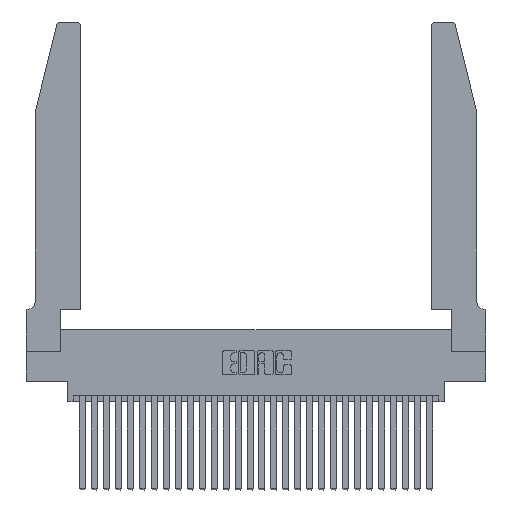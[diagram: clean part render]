
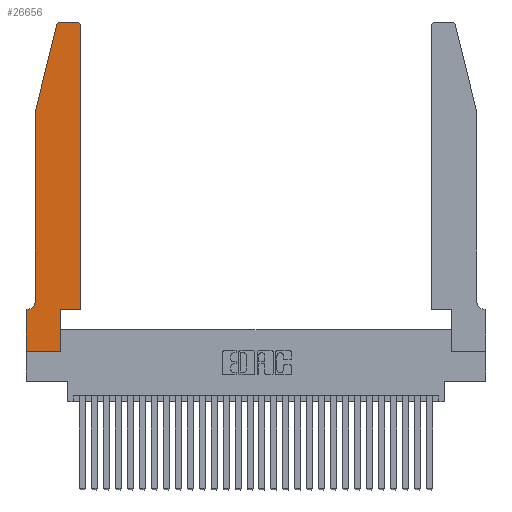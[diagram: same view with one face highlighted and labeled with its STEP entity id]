
A CAD part, top view. The second image highlights one B-rep face of the part: STEP entity #26656.
In plain terms, the highlighted planar face has unit normal (0, 0, 1).
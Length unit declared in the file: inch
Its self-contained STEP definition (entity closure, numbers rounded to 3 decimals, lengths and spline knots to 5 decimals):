
#364 = EDGE_CURVE ( 'NONE', #903, #27673, #7314, .T. ) ;
#465 = EDGE_CURVE ( 'NONE', #7672, #5260, #11283, .T. ) ;
#745 = EDGE_CURVE ( 'NONE', #21035, #6215, #3979, .T. ) ;
#903 = VERTEX_POINT ( 'NONE', #23408 ) ;
#988 = CARTESIAN_POINT ( 'NONE',  ( 0.2865, 0.35, 0.37 ) ) ;
#993 = ORIENTED_EDGE ( 'NONE', *, *, #465, .T. ) ;
#1181 = CARTESIAN_POINT ( 'NONE',  ( 0.284, 2.75, 0.37 ) ) ;
#1803 = VERTEX_POINT ( 'NONE', #988 ) ;
#3058 = ORIENTED_EDGE ( 'NONE', *, *, #11042, .T. ) ;
#3334 = DIRECTION ( 'NONE',  ( 0., 1., 0. ) ) ;
#3357 = VECTOR ( 'NONE', #7024, 39.37008 ) ;
#3956 = LINE ( 'NONE', #26700, #15521 ) ;
#3979 = CIRCLE ( 'NONE', #16523, 0.07 ) ;
#4282 = EDGE_CURVE ( 'NONE', #27673, #25300, #12875, .T. ) ;
#4645 = CARTESIAN_POINT ( 'NONE',  ( 0.0755, 0.35, 0.37 ) ) ;
#4659 = DIRECTION ( 'NONE',  ( 0., -1., 0. ) ) ;
#5152 = CARTESIAN_POINT ( 'NONE',  ( 0.2605, 2.75, 0.37 ) ) ;
#5260 = VERTEX_POINT ( 'NONE', #17508 ) ;
#5823 = ORIENTED_EDGE ( 'NONE', *, *, #745, .T. ) ;
#5982 = CARTESIAN_POINT ( 'NONE',  ( 0., 0.35, 0.37 ) ) ;
#6109 = AXIS2_PLACEMENT_3D ( 'NONE', #13841, #29813, #16131 ) ;
#6215 = VERTEX_POINT ( 'NONE', #25968 ) ;
#6799 = CARTESIAN_POINT ( 'NONE',  ( 0., 0., 0.37 ) ) ;
#6894 = CARTESIAN_POINT ( 'NONE',  ( 0.0755, 2., 0.37 ) ) ;
#6942 = CARTESIAN_POINT ( 'NONE',  ( 0., 0., 0.37 ) ) ;
#7024 = DIRECTION ( 'NONE',  ( -1., 0., 0. ) ) ;
#7314 = LINE ( 'NONE', #5152, #18761 ) ;
#7599 = EDGE_CURVE ( 'NONE', #1803, #7672, #29880, .T. ) ;
#7672 = VERTEX_POINT ( 'NONE', #17500 ) ;
#7917 = CARTESIAN_POINT ( 'NONE',  ( 0.4505, 0.35, 0.37 ) ) ;
#8115 = DIRECTION ( 'NONE',  ( 1., 0., 0. ) ) ;
#8270 = DIRECTION ( 'NONE',  ( -1., 0., 0. ) ) ;
#8468 = CARTESIAN_POINT ( 'NONE',  ( 0., 0.35, 0.37 ) ) ;
#8914 = ORIENTED_EDGE ( 'NONE', *, *, #18953, .T. ) ;
#9139 = DIRECTION ( 'NONE',  ( 1., 0., 0. ) ) ;
#9542 = LINE ( 'NONE', #26634, #20954 ) ;
#10352 = LINE ( 'NONE', #6894, #15696 ) ;
#10544 = VERTEX_POINT ( 'NONE', #25743 ) ;
#10766 = PLANE ( 'NONE',  #27533 ) ;
#11042 = EDGE_CURVE ( 'NONE', #16446, #21035, #10352, .T. ) ;
#11283 = LINE ( 'NONE', #12787, #22721 ) ;
#11735 = CARTESIAN_POINT ( 'NONE',  ( 0., 0., 0.37 ) ) ;
#11928 = VECTOR ( 'NONE', #4659, 39.37008 ) ;
#11986 = DIRECTION ( 'NONE',  ( 0., 0., 1. ) ) ;
#12025 = ORIENTED_EDGE ( 'NONE', *, *, #4282, .T. ) ;
#12452 = EDGE_CURVE ( 'NONE', #10544, #1803, #9542, .T. ) ;
#12787 = CARTESIAN_POINT ( 'NONE',  ( 0.4505, 0.35, 0.37 ) ) ;
#12875 = CIRCLE ( 'NONE', #29224, 0.03 ) ;
#12908 = VERTEX_POINT ( 'NONE', #5982 ) ;
#13841 = CARTESIAN_POINT ( 'NONE',  ( 0.4205, 2.72, 0.37 ) ) ;
#14161 = EDGE_LOOP ( 'NONE', ( #25525, #12025, #8914, #3058, #5823, #25791, #28567, #24692, #18453, #15495, #993, #15075 ) ) ;
#14950 = VERTEX_POINT ( 'NONE', #11735 ) ;
#15075 = ORIENTED_EDGE ( 'NONE', *, *, #15935, .T. ) ;
#15359 = DIRECTION ( 'NONE',  ( 1., 0., 0. ) ) ;
#15495 = ORIENTED_EDGE ( 'NONE', *, *, #7599, .T. ) ;
#15521 = VECTOR ( 'NONE', #24510, 39.37008 ) ;
#15696 = VECTOR ( 'NONE', #20601, 39.37008 ) ;
#15935 = EDGE_CURVE ( 'NONE', #5260, #903, #28627, .T. ) ;
#16131 = DIRECTION ( 'NONE',  ( 1., 0., 0. ) ) ;
#16446 = VERTEX_POINT ( 'NONE', #20488 ) ;
#16515 = LINE ( 'NONE', #6799, #21907 ) ;
#16523 = AXIS2_PLACEMENT_3D ( 'NONE', #21186, #18158, #17938 ) ;
#17500 = CARTESIAN_POINT ( 'NONE',  ( 0.4505, 0.35, 0.37 ) ) ;
#17508 = CARTESIAN_POINT ( 'NONE',  ( 0.4505, 2.72, 0.37 ) ) ;
#17668 = FACE_OUTER_BOUND ( 'NONE', #14161, .T. ) ;
#17720 = VECTOR ( 'NONE', #8115, 39.37008 ) ;
#17938 = DIRECTION ( 'NONE',  ( -1., 0., 0. ) ) ;
#17991 = LINE ( 'NONE', #6942, #11928 ) ;
#18158 = DIRECTION ( 'NONE',  ( 0., 0., -1. ) ) ;
#18453 = ORIENTED_EDGE ( 'NONE', *, *, #12452, .T. ) ;
#18761 = VECTOR ( 'NONE', #8270, 39.37008 ) ;
#18953 = EDGE_CURVE ( 'NONE', #25300, #16446, #3956, .T. ) ;
#20488 = CARTESIAN_POINT ( 'NONE',  ( 0.0755, 2., 0.37 ) ) ;
#20601 = DIRECTION ( 'NONE',  ( 0., -1., 0. ) ) ;
#20954 = VECTOR ( 'NONE', #28916, 39.37008 ) ;
#21035 = VERTEX_POINT ( 'NONE', #26102 ) ;
#21186 = CARTESIAN_POINT ( 'NONE',  ( 0.0055, 0.42, 0.37 ) ) ;
#21907 = VECTOR ( 'NONE', #9139, 39.37008 ) ;
#22721 = VECTOR ( 'NONE', #3334, 39.37008 ) ;
#23408 = CARTESIAN_POINT ( 'NONE',  ( 0.4205, 2.75, 0.37 ) ) ;
#24510 = DIRECTION ( 'NONE',  ( -0.239, -0.971, 0. ) ) ;
#24692 = ORIENTED_EDGE ( 'NONE', *, *, #28543, .T. ) ;
#24974 = EDGE_CURVE ( 'NONE', #6215, #12908, #27083, .T. ) ;
#25300 = VERTEX_POINT ( 'NONE', #26522 ) ;
#25525 = ORIENTED_EDGE ( 'NONE', *, *, #364, .T. ) ;
#25677 = CARTESIAN_POINT ( 'NONE',  ( 0.284, 2.72, 0.37 ) ) ;
#25743 = CARTESIAN_POINT ( 'NONE',  ( 0.2865, 0., 0.37 ) ) ;
#25791 = ORIENTED_EDGE ( 'NONE', *, *, #24974, .T. ) ;
#25968 = CARTESIAN_POINT ( 'NONE',  ( 0.0055, 0.35, 0.37 ) ) ;
#26102 = CARTESIAN_POINT ( 'NONE',  ( 0.0755, 0.42, 0.37 ) ) ;
#26522 = CARTESIAN_POINT ( 'NONE',  ( 0.25487, 2.72718, 0.37 ) ) ;
#26634 = CARTESIAN_POINT ( 'NONE',  ( 0.2865, 0.35, 0.37 ) ) ;
#26656 = ADVANCED_FACE ( 'NONE', ( #17668 ), #10766, .T. ) ;
#26700 = CARTESIAN_POINT ( 'NONE',  ( 0.0755, 2., 0.37 ) ) ;
#27083 = LINE ( 'NONE', #4645, #3357 ) ;
#27533 = AXIS2_PLACEMENT_3D ( 'NONE', #8468, #29037, #15359 ) ;
#27673 = VERTEX_POINT ( 'NONE', #1181 ) ;
#27951 = DIRECTION ( 'NONE',  ( 1., 0., 0. ) ) ;
#28009 = EDGE_CURVE ( 'NONE', #12908, #14950, #17991, .T. ) ;
#28543 = EDGE_CURVE ( 'NONE', #14950, #10544, #16515, .T. ) ;
#28567 = ORIENTED_EDGE ( 'NONE', *, *, #28009, .T. ) ;
#28627 = CIRCLE ( 'NONE', #6109, 0.03 ) ;
#28916 = DIRECTION ( 'NONE',  ( 0., 1., 0. ) ) ;
#29037 = DIRECTION ( 'NONE',  ( 0., 0., 1. ) ) ;
#29224 = AXIS2_PLACEMENT_3D ( 'NONE', #25677, #11986, #27951 ) ;
#29813 = DIRECTION ( 'NONE',  ( 0., 0., 1. ) ) ;
#29880 = LINE ( 'NONE', #7917, #17720 ) ;
